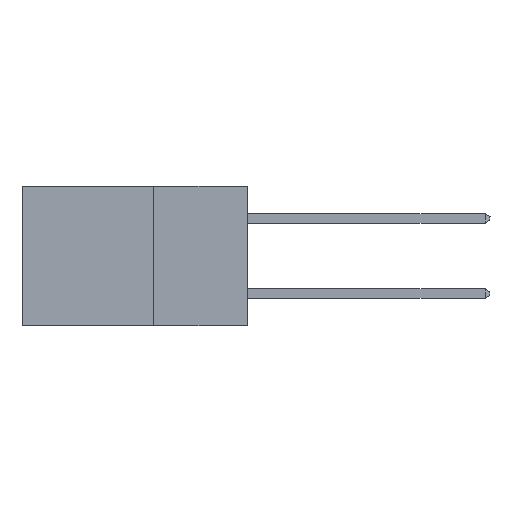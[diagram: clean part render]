
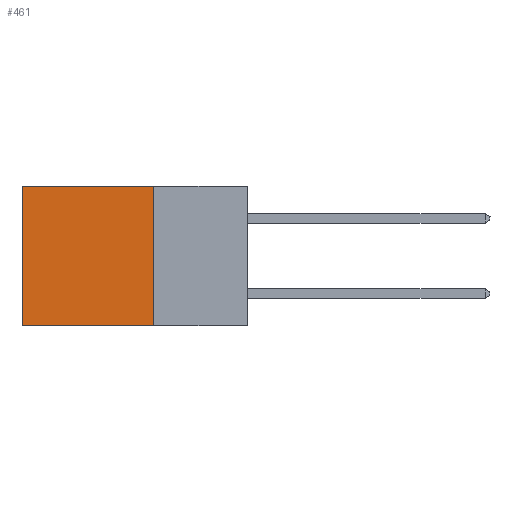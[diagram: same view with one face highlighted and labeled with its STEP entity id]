
A CAD part, left-side view. The second image highlights one B-rep face of the part: STEP entity #461.
In plain terms, the highlighted planar face has unit normal (-1, 0, 0).
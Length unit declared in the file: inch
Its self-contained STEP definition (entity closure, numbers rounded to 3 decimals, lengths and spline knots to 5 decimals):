
#246 = ORIENTED_EDGE ( 'NONE', *, *, #12423, .T. ) ;
#428 = VERTEX_POINT ( 'NONE', #16517 ) ;
#461 = ADVANCED_FACE ( 'NONE', ( #5433 ), #9789, .F. ) ;
#614 = ORIENTED_EDGE ( 'NONE', *, *, #6646, .T. ) ;
#1643 = LINE ( 'NONE', #6207, #10073 ) ;
#1734 = CARTESIAN_POINT ( 'NONE',  ( 0.2615, 0.6, -0.37 ) ) ;
#2047 = VERTEX_POINT ( 'NONE', #1734 ) ;
#3269 = CARTESIAN_POINT ( 'NONE',  ( 0.2615, 0.25, -0.37 ) ) ;
#3443 = CARTESIAN_POINT ( 'NONE',  ( 0.2615, 0.6, 0. ) ) ;
#4055 = LINE ( 'NONE', #16597, #13113 ) ;
#4466 = DIRECTION ( 'NONE',  ( 0., 1., 0. ) ) ;
#5433 = FACE_OUTER_BOUND ( 'NONE', #14681, .T. ) ;
#6207 = CARTESIAN_POINT ( 'NONE',  ( 0.2615, 0.25, -0.37 ) ) ;
#6270 = VECTOR ( 'NONE', #9761, 39.37008 ) ;
#6646 = EDGE_CURVE ( 'NONE', #11479, #2047, #16653, .T. ) ;
#8255 = CARTESIAN_POINT ( 'NONE',  ( 0.2615, 0.6, -0.37 ) ) ;
#8700 = LINE ( 'NONE', #3269, #14716 ) ;
#9325 = ORIENTED_EDGE ( 'NONE', *, *, #10334, .F. ) ;
#9761 = DIRECTION ( 'NONE',  ( 0., 0., -1. ) ) ;
#9789 = PLANE ( 'NONE',  #12115 ) ;
#10073 = VECTOR ( 'NONE', #4466, 39.37008 ) ;
#10310 = EDGE_CURVE ( 'NONE', #11655, #2047, #1643, .T. ) ;
#10334 = EDGE_CURVE ( 'NONE', #428, #11655, #8700, .T. ) ;
#10608 = ORIENTED_EDGE ( 'NONE', *, *, #10310, .F. ) ;
#11145 = DIRECTION ( 'NONE',  ( 0., 1., 0. ) ) ;
#11479 = VERTEX_POINT ( 'NONE', #3443 ) ;
#11655 = VERTEX_POINT ( 'NONE', #13007 ) ;
#12115 = AXIS2_PLACEMENT_3D ( 'NONE', #13773, #15316, #12487 ) ;
#12423 = EDGE_CURVE ( 'NONE', #428, #11479, #4055, .T. ) ;
#12487 = DIRECTION ( 'NONE',  ( 0., 0., -1. ) ) ;
#12925 = DIRECTION ( 'NONE',  ( 0., 0., -1. ) ) ;
#13007 = CARTESIAN_POINT ( 'NONE',  ( 0.2615, 0.25, -0.37 ) ) ;
#13113 = VECTOR ( 'NONE', #11145, 39.37008 ) ;
#13773 = CARTESIAN_POINT ( 'NONE',  ( 0.2615, 0.25, -0.37 ) ) ;
#14681 = EDGE_LOOP ( 'NONE', ( #614, #10608, #9325, #246 ) ) ;
#14716 = VECTOR ( 'NONE', #12925, 39.37008 ) ;
#15316 = DIRECTION ( 'NONE',  ( 1., 0., 0. ) ) ;
#16517 = CARTESIAN_POINT ( 'NONE',  ( 0.2615, 0.25, 0. ) ) ;
#16597 = CARTESIAN_POINT ( 'NONE',  ( 0.2615, 0.25, 0. ) ) ;
#16653 = LINE ( 'NONE', #8255, #6270 ) ;
